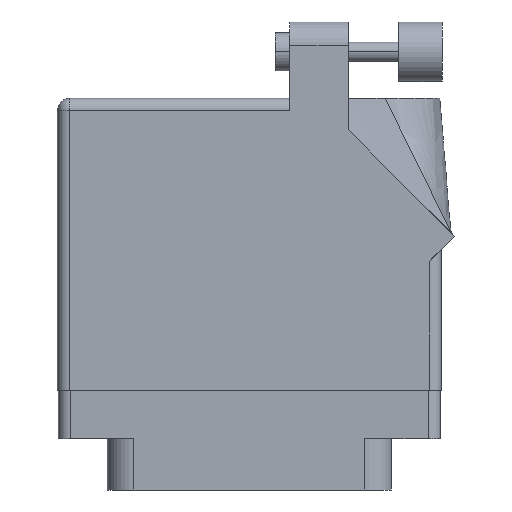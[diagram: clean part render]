
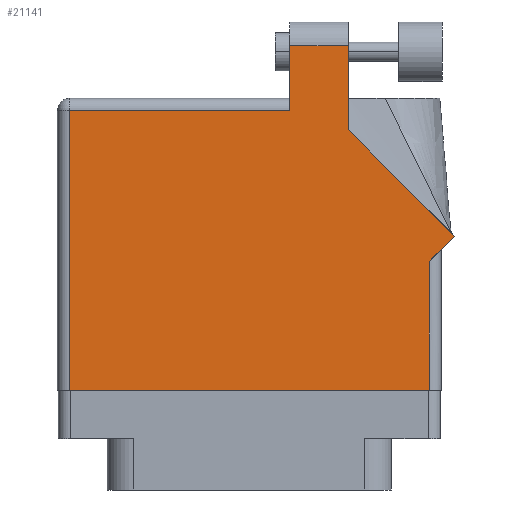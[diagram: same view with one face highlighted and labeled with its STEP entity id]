
A CAD part, front view. The second image highlights one B-rep face of the part: STEP entity #21141.
In plain terms, the highlighted face is planar.
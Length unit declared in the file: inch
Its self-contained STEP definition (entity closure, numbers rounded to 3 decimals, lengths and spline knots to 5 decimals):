
#148 = CARTESIAN_POINT ( 'NONE',  ( 0.519, 1.26442, 0.455 ) ) ;
#909 = VERTEX_POINT ( 'NONE', #13779 ) ;
#1164 = LINE ( 'NONE', #4261, #28771 ) ;
#2964 = LINE ( 'NONE', #13486, #20373 ) ;
#3309 = EDGE_CURVE ( 'NONE', #15565, #39714, #12498, .T. ) ;
#3396 = VECTOR ( 'NONE', #26824, 39.37008 ) ;
#3797 = ORIENTED_EDGE ( 'NONE', *, *, #27128, .T. ) ;
#3925 = VECTOR ( 'NONE', #16635, 39.37008 ) ;
#4261 = CARTESIAN_POINT ( 'NONE',  ( 0.212, 1.705, 0.455 ) ) ;
#4678 = ORIENTED_EDGE ( 'NONE', *, *, #17596, .T. ) ;
#5044 = CARTESIAN_POINT ( 'NONE',  ( 0.943, 0.637, 0.455 ) ) ;
#5847 = FACE_OUTER_BOUND ( 'NONE', #30175, .T. ) ;
#6050 = CARTESIAN_POINT ( 'NONE',  ( -0.943, 1.368, 0.455 ) ) ;
#6471 = EDGE_CURVE ( 'NONE', #26981, #909, #35569, .T. ) ;
#7355 = LINE ( 'NONE', #37721, #17530 ) ;
#7374 = VECTOR ( 'NONE', #37249, 39.37008 ) ;
#7418 = EDGE_CURVE ( 'NONE', #32872, #26981, #1164, .T. ) ;
#7490 = VECTOR ( 'NONE', #20956, 39.37008 ) ;
#8105 = PLANE ( 'NONE',  #26186 ) ;
#8568 = VERTEX_POINT ( 'NONE', #31631 ) ;
#9401 = LINE ( 'NONE', #31635, #10362 ) ;
#10362 = VECTOR ( 'NONE', #12652, 39.37008 ) ;
#12498 = LINE ( 'NONE', #19483, #13942 ) ;
#12588 = LINE ( 'NONE', #19334, #3925 ) ;
#12652 = DIRECTION ( 'NONE',  ( 1., 0., 0. ) ) ;
#13486 = CARTESIAN_POINT ( 'NONE',  ( -1.005, 1.368, 0.455 ) ) ;
#13649 = DIRECTION ( 'NONE',  ( -0.707, 0.707, 0. ) ) ;
#13779 = CARTESIAN_POINT ( 'NONE',  ( 0.212, 1.368, 0.455 ) ) ;
#13942 = VECTOR ( 'NONE', #13649, 39.37008 ) ;
#14531 = LINE ( 'NONE', #5044, #3396 ) ;
#15565 = VERTEX_POINT ( 'NONE', #21512 ) ;
#16502 = VERTEX_POINT ( 'NONE', #24677 ) ;
#16635 = DIRECTION ( 'NONE',  ( 0.707, 0.707, 0. ) ) ;
#17530 = VECTOR ( 'NONE', #24723, 39.37008 ) ;
#17596 = EDGE_CURVE ( 'NONE', #8568, #19039, #9401, .T. ) ;
#17720 = ORIENTED_EDGE ( 'NONE', *, *, #33987, .T. ) ;
#18000 = CARTESIAN_POINT ( 'NONE',  ( 0.212, 1.43, 0.455 ) ) ;
#19039 = VERTEX_POINT ( 'NONE', #38991 ) ;
#19334 = CARTESIAN_POINT ( 'NONE',  ( 1.005, 0.637, 0.455 ) ) ;
#19483 = CARTESIAN_POINT ( 'NONE',  ( 1.07571, 0.70771, 0.455 ) ) ;
#20049 = CARTESIAN_POINT ( 'NONE',  ( 0.212, 1.705, 0.455 ) ) ;
#20352 = EDGE_CURVE ( 'NONE', #39714, #32872, #21350, .T. ) ;
#20373 = VECTOR ( 'NONE', #35179, 39.37008 ) ;
#20956 = DIRECTION ( 'NONE',  ( 0., -1., 0. ) ) ;
#21141 = ADVANCED_FACE ( 'NONE', ( #5847 ), #8105, .F. ) ;
#21350 = LINE ( 'NONE', #39966, #7374 ) ;
#21512 = CARTESIAN_POINT ( 'NONE',  ( 1.07571, 0.70771, 0.455 ) ) ;
#21683 = ORIENTED_EDGE ( 'NONE', *, *, #20352, .T. ) ;
#23672 = DIRECTION ( 'NONE',  ( -1., 0., 0. ) ) ;
#24049 = ORIENTED_EDGE ( 'NONE', *, *, #33996, .T. ) ;
#24070 = VERTEX_POINT ( 'NONE', #6050 ) ;
#24677 = CARTESIAN_POINT ( 'NONE',  ( 0.943, 0.575, 0.455 ) ) ;
#24723 = DIRECTION ( 'NONE',  ( 0., -1., 0. ) ) ;
#25655 = ORIENTED_EDGE ( 'NONE', *, *, #25778, .T. ) ;
#25778 = EDGE_CURVE ( 'NONE', #24070, #8568, #7355, .T. ) ;
#25916 = DIRECTION ( 'NONE',  ( -1., 0., 0. ) ) ;
#26186 = AXIS2_PLACEMENT_3D ( 'NONE', #29758, #38956, #23672 ) ;
#26824 = DIRECTION ( 'NONE',  ( 0., 1., 0. ) ) ;
#26981 = VERTEX_POINT ( 'NONE', #20049 ) ;
#27128 = EDGE_CURVE ( 'NONE', #19039, #16502, #14531, .T. ) ;
#27512 = ORIENTED_EDGE ( 'NONE', *, *, #6471, .T. ) ;
#28771 = VECTOR ( 'NONE', #25916, 39.37008 ) ;
#29758 = CARTESIAN_POINT ( 'NONE',  ( -1.005, 1.43, 0.455 ) ) ;
#29913 = ORIENTED_EDGE ( 'NONE', *, *, #3309, .T. ) ;
#30175 = EDGE_LOOP ( 'NONE', ( #21683, #32225, #27512, #17720, #25655, #4678, #3797, #24049, #29913 ) ) ;
#31631 = CARTESIAN_POINT ( 'NONE',  ( -0.943, -0.1, 0.455 ) ) ;
#31635 = CARTESIAN_POINT ( 'NONE',  ( -1.005, -0.1, 0.455 ) ) ;
#32225 = ORIENTED_EDGE ( 'NONE', *, *, #7418, .T. ) ;
#32872 = VERTEX_POINT ( 'NONE', #37077 ) ;
#33987 = EDGE_CURVE ( 'NONE', #909, #24070, #2964, .T. ) ;
#33996 = EDGE_CURVE ( 'NONE', #16502, #15565, #12588, .T. ) ;
#35179 = DIRECTION ( 'NONE',  ( -1., 0., 0. ) ) ;
#35569 = LINE ( 'NONE', #18000, #7490 ) ;
#37077 = CARTESIAN_POINT ( 'NONE',  ( 0.519, 1.705, 0.455 ) ) ;
#37249 = DIRECTION ( 'NONE',  ( 0., 1., 0. ) ) ;
#37721 = CARTESIAN_POINT ( 'NONE',  ( -0.943, -0.1, 0.455 ) ) ;
#38956 = DIRECTION ( 'NONE',  ( 0., 0., -1. ) ) ;
#38991 = CARTESIAN_POINT ( 'NONE',  ( 0.943, -0.1, 0.455 ) ) ;
#39714 = VERTEX_POINT ( 'NONE', #148 ) ;
#39966 = CARTESIAN_POINT ( 'NONE',  ( 0.519, 1.26442, 0.455 ) ) ;
